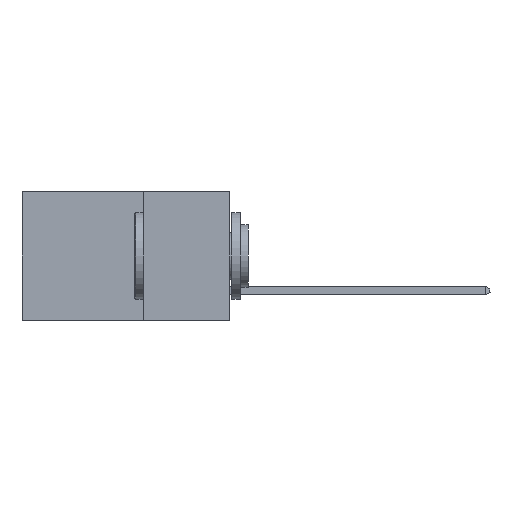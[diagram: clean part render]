
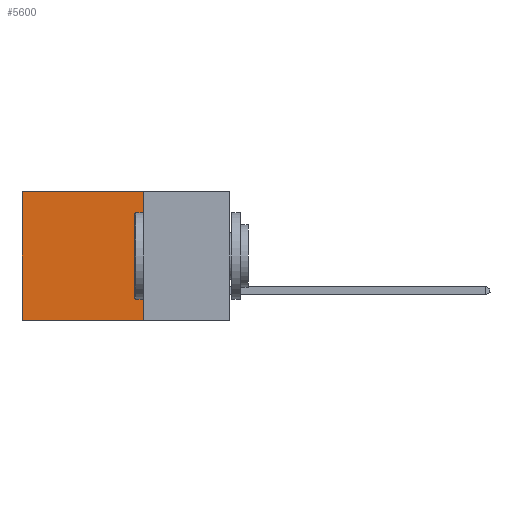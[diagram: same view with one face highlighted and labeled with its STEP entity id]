
A CAD part, left-side view. The second image highlights one B-rep face of the part: STEP entity #5600.
In plain terms, the highlighted planar face has unit normal (-1, 0, 0).
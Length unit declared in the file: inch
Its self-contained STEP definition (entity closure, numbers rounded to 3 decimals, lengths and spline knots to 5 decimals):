
#84 = DIRECTION ( 'NONE',  ( 1., 0., 0. ) ) ;
#179 = LINE ( 'NONE', #7492, #11742 ) ;
#254 = EDGE_CURVE ( 'NONE', #4483, #7967, #278, .T. ) ;
#278 = LINE ( 'NONE', #7223, #11208 ) ;
#393 = CARTESIAN_POINT ( 'NONE',  ( 0.298, 0.25, -0.37 ) ) ;
#748 = DIRECTION ( 'NONE',  ( 0., 1., 0. ) ) ;
#1780 = DIRECTION ( 'NONE',  ( 0., 0., -1. ) ) ;
#2043 = DIRECTION ( 'NONE',  ( 0., 0., -1. ) ) ;
#2103 = ORIENTED_EDGE ( 'NONE', *, *, #254, .T. ) ;
#3222 = VERTEX_POINT ( 'NONE', #8824 ) ;
#3524 = CARTESIAN_POINT ( 'NONE',  ( 0.298, 0.25, 0. ) ) ;
#4197 = LINE ( 'NONE', #393, #9672 ) ;
#4483 = VERTEX_POINT ( 'NONE', #11316 ) ;
#4575 = CARTESIAN_POINT ( 'NONE',  ( 0.298, 0.6, -0.37 ) ) ;
#4618 = ORIENTED_EDGE ( 'NONE', *, *, #8235, .T. ) ;
#4909 = AXIS2_PLACEMENT_3D ( 'NONE', #11138, #84, #8786 ) ;
#5215 = CARTESIAN_POINT ( 'NONE',  ( 0.298, 0.25, 0. ) ) ;
#5600 = ADVANCED_FACE ( 'NONE', ( #11570 ), #6579, .F. ) ;
#5930 = DIRECTION ( 'NONE',  ( 0., 1., 0. ) ) ;
#6579 = PLANE ( 'NONE',  #4909 ) ;
#7223 = CARTESIAN_POINT ( 'NONE',  ( 0.298, 0.6, 0. ) ) ;
#7379 = EDGE_CURVE ( 'NONE', #3222, #7967, #4197, .T. ) ;
#7492 = CARTESIAN_POINT ( 'NONE',  ( 0.298, 0.25, 0. ) ) ;
#7967 = VERTEX_POINT ( 'NONE', #4575 ) ;
#7970 = LINE ( 'NONE', #5215, #9998 ) ;
#8235 = EDGE_CURVE ( 'NONE', #8809, #4483, #7970, .T. ) ;
#8786 = DIRECTION ( 'NONE',  ( 0., 0., -1. ) ) ;
#8809 = VERTEX_POINT ( 'NONE', #3524 ) ;
#8824 = CARTESIAN_POINT ( 'NONE',  ( 0.298, 0.25, -0.37 ) ) ;
#9672 = VECTOR ( 'NONE', #5930, 39.37008 ) ;
#9998 = VECTOR ( 'NONE', #748, 39.37008 ) ;
#10220 = ORIENTED_EDGE ( 'NONE', *, *, #12077, .F. ) ;
#11138 = CARTESIAN_POINT ( 'NONE',  ( 0.298, 0.25, 0. ) ) ;
#11208 = VECTOR ( 'NONE', #1780, 39.37008 ) ;
#11316 = CARTESIAN_POINT ( 'NONE',  ( 0.298, 0.6, 0. ) ) ;
#11570 = FACE_OUTER_BOUND ( 'NONE', #11617, .T. ) ;
#11617 = EDGE_LOOP ( 'NONE', ( #2103, #13445, #10220, #4618 ) ) ;
#11742 = VECTOR ( 'NONE', #2043, 39.37008 ) ;
#12077 = EDGE_CURVE ( 'NONE', #8809, #3222, #179, .T. ) ;
#13445 = ORIENTED_EDGE ( 'NONE', *, *, #7379, .F. ) ;
